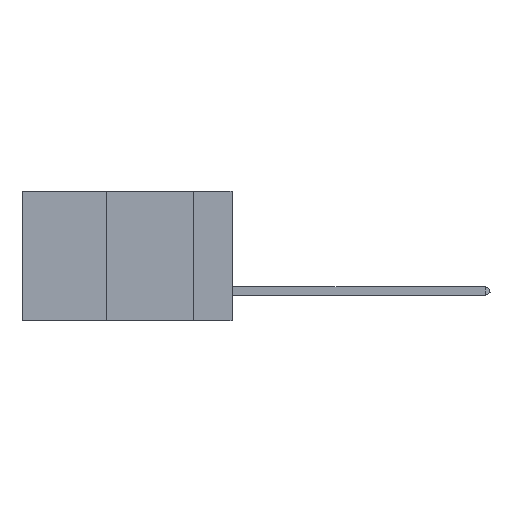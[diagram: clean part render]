
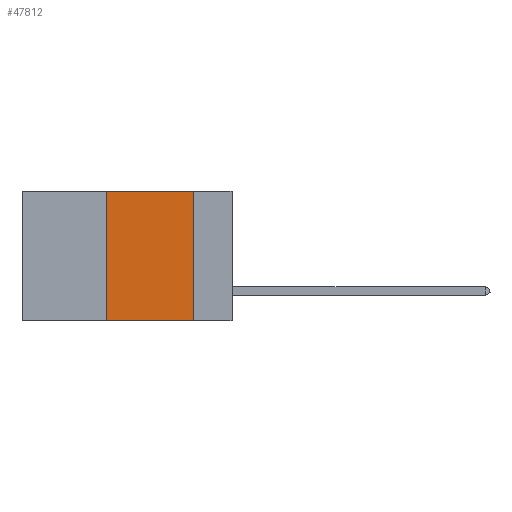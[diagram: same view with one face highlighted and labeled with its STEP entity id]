
A CAD part, left-side view. The second image highlights one B-rep face of the part: STEP entity #47812.
In plain terms, the highlighted planar face has unit normal (-1, 0, 0).
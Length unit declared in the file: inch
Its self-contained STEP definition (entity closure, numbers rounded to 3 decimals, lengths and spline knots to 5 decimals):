
#299 = DIRECTION ( 'NONE',  ( 0., -1., 0. ) ) ;
#1599 = LINE ( 'NONE', #31778, #37859 ) ;
#1912 = VECTOR ( 'NONE', #299, 39.37008 ) ;
#3903 = PLANE ( 'NONE',  #33848 ) ;
#5876 = CARTESIAN_POINT ( 'NONE',  ( 0., 0.11, -0.37 ) ) ;
#7646 = VECTOR ( 'NONE', #35658, 39.37008 ) ;
#9145 = VECTOR ( 'NONE', #15189, 39.37008 ) ;
#10010 = ORIENTED_EDGE ( 'NONE', *, *, #26937, .F. ) ;
#13592 = CARTESIAN_POINT ( 'NONE',  ( 0., 0.36, -0.37 ) ) ;
#15189 = DIRECTION ( 'NONE',  ( 0., 0., -1. ) ) ;
#17581 = EDGE_LOOP ( 'NONE', ( #21760, #10010, #48171, #38400 ) ) ;
#18006 = LINE ( 'NONE', #43263, #7646 ) ;
#19080 = VERTEX_POINT ( 'NONE', #13592 ) ;
#19847 = DIRECTION ( 'NONE',  ( 1., 0., 0. ) ) ;
#19990 = DIRECTION ( 'NONE',  ( 0., -1., 0. ) ) ;
#21760 = ORIENTED_EDGE ( 'NONE', *, *, #39426, .F. ) ;
#22432 = VERTEX_POINT ( 'NONE', #5876 ) ;
#26937 = EDGE_CURVE ( 'NONE', #48634, #43606, #28494, .T. ) ;
#28494 = LINE ( 'NONE', #46938, #1912 ) ;
#30873 = CARTESIAN_POINT ( 'NONE',  ( 0., 0.11, 0. ) ) ;
#31778 = CARTESIAN_POINT ( 'NONE',  ( 0., 0.6, -0.37 ) ) ;
#33848 = AXIS2_PLACEMENT_3D ( 'NONE', #38887, #19847, #38562 ) ;
#34632 = LINE ( 'NONE', #30873, #9145 ) ;
#35658 = DIRECTION ( 'NONE',  ( 0., 0., 1. ) ) ;
#36812 = EDGE_CURVE ( 'NONE', #19080, #22432, #1599, .T. ) ;
#36823 = EDGE_CURVE ( 'NONE', #19080, #48634, #18006, .T. ) ;
#37859 = VECTOR ( 'NONE', #19990, 39.37008 ) ;
#38400 = ORIENTED_EDGE ( 'NONE', *, *, #36812, .T. ) ;
#38562 = DIRECTION ( 'NONE',  ( 0., 0., -1. ) ) ;
#38887 = CARTESIAN_POINT ( 'NONE',  ( 0., 0.6, 0. ) ) ;
#39425 = CARTESIAN_POINT ( 'NONE',  ( 0., 0.11, 0. ) ) ;
#39426 = EDGE_CURVE ( 'NONE', #43606, #22432, #34632, .T. ) ;
#41105 = FACE_OUTER_BOUND ( 'NONE', #17581, .T. ) ;
#43263 = CARTESIAN_POINT ( 'NONE',  ( 0., 0.36, 0. ) ) ;
#43606 = VERTEX_POINT ( 'NONE', #39425 ) ;
#46403 = CARTESIAN_POINT ( 'NONE',  ( 0., 0.36, 0. ) ) ;
#46938 = CARTESIAN_POINT ( 'NONE',  ( 0., 0.6, 0. ) ) ;
#47812 = ADVANCED_FACE ( 'NONE', ( #41105 ), #3903, .F. ) ;
#48171 = ORIENTED_EDGE ( 'NONE', *, *, #36823, .F. ) ;
#48634 = VERTEX_POINT ( 'NONE', #46403 ) ;
